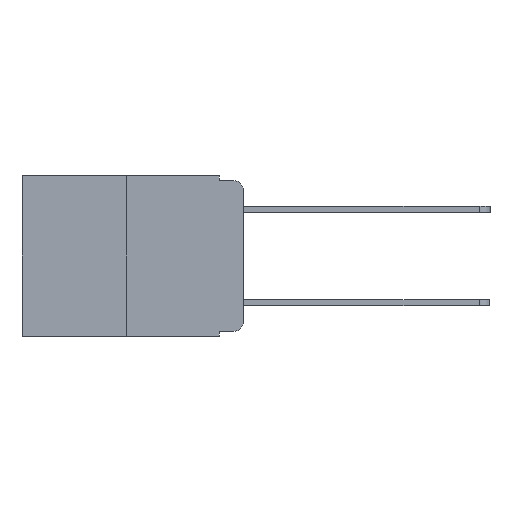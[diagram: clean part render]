
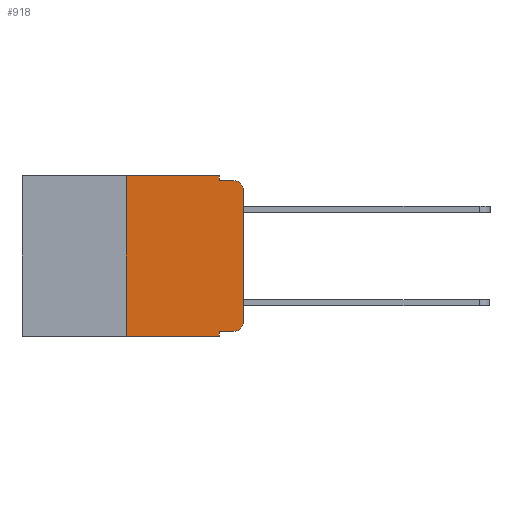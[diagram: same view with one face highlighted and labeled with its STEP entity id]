
A CAD part, left-side view. The second image highlights one B-rep face of the part: STEP entity #918.
In plain terms, the highlighted planar face has unit normal (-1, 0, 0).
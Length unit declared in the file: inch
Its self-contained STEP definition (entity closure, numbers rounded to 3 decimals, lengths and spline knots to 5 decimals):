
#275 = DIRECTION ( 'NONE',  ( 1., 0., 0. ) ) ;
#280 = DIRECTION ( 'NONE',  ( 0., 0., -1. ) ) ;
#358 = VERTEX_POINT ( 'NONE', #8227 ) ;
#691 = VECTOR ( 'NONE', #16687, 39.37008 ) ;
#780 = LINE ( 'NONE', #6265, #15321 ) ;
#918 = ADVANCED_FACE ( 'NONE', ( #2012 ), #3815, .F. ) ;
#939 = DIRECTION ( 'NONE',  ( -1., 0., 0. ) ) ;
#952 = CARTESIAN_POINT ( 'NONE',  ( 0., 0.25, -0.343 ) ) ;
#1030 = ORIENTED_EDGE ( 'NONE', *, *, #13807, .T. ) ;
#1103 = ORIENTED_EDGE ( 'NONE', *, *, #17932, .F. ) ;
#1312 = LINE ( 'NONE', #16135, #4655 ) ;
#1351 = ORIENTED_EDGE ( 'NONE', *, *, #1771, .F. ) ;
#1380 = EDGE_CURVE ( 'NONE', #13575, #15057, #2000, .T. ) ;
#1771 = EDGE_CURVE ( 'NONE', #9628, #3208, #10822, .T. ) ;
#1981 = ORIENTED_EDGE ( 'NONE', *, *, #15716, .F. ) ;
#2000 = CIRCLE ( 'NONE', #6870, 0.02 ) ;
#2012 = FACE_OUTER_BOUND ( 'NONE', #2747, .T. ) ;
#2114 = LINE ( 'NONE', #11918, #12963 ) ;
#2508 = CARTESIAN_POINT ( 'NONE',  ( 0., 0., -0.03 ) ) ;
#2587 = ORIENTED_EDGE ( 'NONE', *, *, #5270, .T. ) ;
#2642 = CARTESIAN_POINT ( 'NONE',  ( 0., 0.25, 0. ) ) ;
#2747 = EDGE_LOOP ( 'NONE', ( #2587, #11738, #8355, #1103, #1981, #16691, #3247, #1351, #1030, #5750 ) ) ;
#2771 = DIRECTION ( 'NONE',  ( -1., 0., 0. ) ) ;
#3208 = VERTEX_POINT ( 'NONE', #15648 ) ;
#3247 = ORIENTED_EDGE ( 'NONE', *, *, #10072, .T. ) ;
#3268 = VECTOR ( 'NONE', #12088, 39.37008 ) ;
#3815 = PLANE ( 'NONE',  #13036 ) ;
#4494 = LINE ( 'NONE', #2642, #691 ) ;
#4655 = VECTOR ( 'NONE', #6303, 39.37008 ) ;
#5158 = LINE ( 'NONE', #5769, #12239 ) ;
#5270 = EDGE_CURVE ( 'NONE', #15057, #6321, #5158, .T. ) ;
#5750 = ORIENTED_EDGE ( 'NONE', *, *, #1380, .T. ) ;
#5769 = CARTESIAN_POINT ( 'NONE',  ( 0., 0., 0. ) ) ;
#6265 = CARTESIAN_POINT ( 'NONE',  ( 0., 0.051, -0.01 ) ) ;
#6303 = DIRECTION ( 'NONE',  ( 0., -1., 0. ) ) ;
#6321 = VERTEX_POINT ( 'NONE', #2508 ) ;
#6870 = AXIS2_PLACEMENT_3D ( 'NONE', #17852, #2771, #16809 ) ;
#7564 = CARTESIAN_POINT ( 'NONE',  ( 0., 0.051, 0. ) ) ;
#7974 = CARTESIAN_POINT ( 'NONE',  ( 0., 0.473, 0. ) ) ;
#8077 = CARTESIAN_POINT ( 'NONE',  ( 0., 0.051, -0.333 ) ) ;
#8227 = CARTESIAN_POINT ( 'NONE',  ( 0., 0.02, -0.01 ) ) ;
#8355 = ORIENTED_EDGE ( 'NONE', *, *, #10142, .F. ) ;
#8360 = VERTEX_POINT ( 'NONE', #13506 ) ;
#8432 = LINE ( 'NONE', #7974, #15445 ) ;
#9263 = CARTESIAN_POINT ( 'NONE',  ( 0., 0., -0.313 ) ) ;
#9397 = CARTESIAN_POINT ( 'NONE',  ( 0., 0.02, -0.03 ) ) ;
#9628 = VERTEX_POINT ( 'NONE', #8077 ) ;
#10072 = EDGE_CURVE ( 'NONE', #15739, #3208, #2114, .T. ) ;
#10142 = EDGE_CURVE ( 'NONE', #8360, #358, #780, .T. ) ;
#10178 = DIRECTION ( 'NONE',  ( 0., 0., -1. ) ) ;
#10822 = LINE ( 'NONE', #14187, #18182 ) ;
#10823 = DIRECTION ( 'NONE',  ( 0., 0., -1. ) ) ;
#11354 = CARTESIAN_POINT ( 'NONE',  ( 0., 0.02, -0.333 ) ) ;
#11540 = EDGE_CURVE ( 'NONE', #6321, #358, #13980, .T. ) ;
#11738 = ORIENTED_EDGE ( 'NONE', *, *, #11540, .T. ) ;
#11918 = CARTESIAN_POINT ( 'NONE',  ( 0., 0.473, -0.343 ) ) ;
#12088 = DIRECTION ( 'NONE',  ( 0., 0., -1. ) ) ;
#12239 = VECTOR ( 'NONE', #15588, 39.37008 ) ;
#12320 = EDGE_CURVE ( 'NONE', #15739, #16418, #4494, .T. ) ;
#12963 = VECTOR ( 'NONE', #13328, 39.37008 ) ;
#13036 = AXIS2_PLACEMENT_3D ( 'NONE', #16345, #275, #280 ) ;
#13328 = DIRECTION ( 'NONE',  ( 0., -1., 0. ) ) ;
#13454 = DIRECTION ( 'NONE',  ( 0., -1., 0. ) ) ;
#13506 = CARTESIAN_POINT ( 'NONE',  ( 0., 0.051, -0.01 ) ) ;
#13575 = VERTEX_POINT ( 'NONE', #11354 ) ;
#13716 = CARTESIAN_POINT ( 'NONE',  ( 0., 0.25, 0. ) ) ;
#13807 = EDGE_CURVE ( 'NONE', #9628, #13575, #1312, .T. ) ;
#13980 = CIRCLE ( 'NONE', #16919, 0.02 ) ;
#14187 = CARTESIAN_POINT ( 'NONE',  ( 0., 0.051, 0. ) ) ;
#14952 = VERTEX_POINT ( 'NONE', #7564 ) ;
#15057 = VERTEX_POINT ( 'NONE', #9263 ) ;
#15321 = VECTOR ( 'NONE', #13454, 39.37008 ) ;
#15445 = VECTOR ( 'NONE', #17756, 39.37008 ) ;
#15588 = DIRECTION ( 'NONE',  ( 0., 0., 1. ) ) ;
#15648 = CARTESIAN_POINT ( 'NONE',  ( 0., 0.051, -0.343 ) ) ;
#15716 = EDGE_CURVE ( 'NONE', #16418, #14952, #8432, .T. ) ;
#15739 = VERTEX_POINT ( 'NONE', #952 ) ;
#16135 = CARTESIAN_POINT ( 'NONE',  ( 0., 0.051, -0.333 ) ) ;
#16194 = CARTESIAN_POINT ( 'NONE',  ( 0., 0.051, 0. ) ) ;
#16345 = CARTESIAN_POINT ( 'NONE',  ( 0., 0.473, 0. ) ) ;
#16418 = VERTEX_POINT ( 'NONE', #13716 ) ;
#16687 = DIRECTION ( 'NONE',  ( 0., 0., 1. ) ) ;
#16691 = ORIENTED_EDGE ( 'NONE', *, *, #12320, .F. ) ;
#16809 = DIRECTION ( 'NONE',  ( 0., 0., -1. ) ) ;
#16919 = AXIS2_PLACEMENT_3D ( 'NONE', #9397, #939, #10823 ) ;
#17756 = DIRECTION ( 'NONE',  ( 0., -1., 0. ) ) ;
#17852 = CARTESIAN_POINT ( 'NONE',  ( 0., 0.02, -0.313 ) ) ;
#17932 = EDGE_CURVE ( 'NONE', #14952, #8360, #18136, .T. ) ;
#18136 = LINE ( 'NONE', #16194, #3268 ) ;
#18182 = VECTOR ( 'NONE', #10178, 39.37008 ) ;
